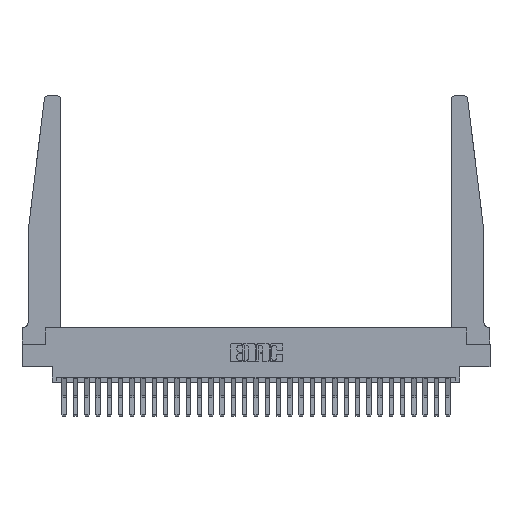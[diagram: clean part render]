
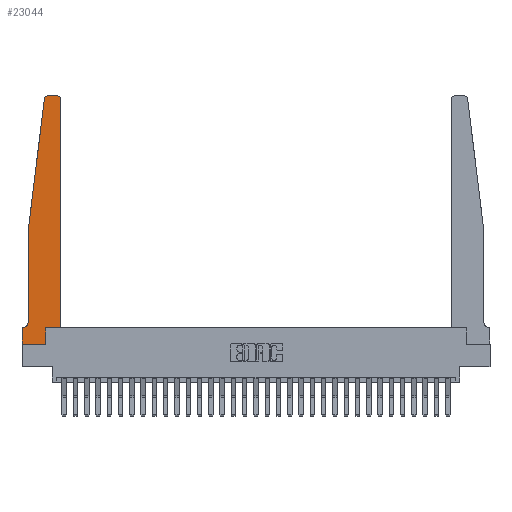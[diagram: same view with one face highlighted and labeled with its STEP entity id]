
A CAD part, top view. The second image highlights one B-rep face of the part: STEP entity #23044.
In plain terms, the highlighted planar face has unit normal (0, 0, 1).
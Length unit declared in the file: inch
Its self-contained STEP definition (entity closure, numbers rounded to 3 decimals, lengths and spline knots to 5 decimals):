
#455 = CARTESIAN_POINT ( 'NONE',  ( 0., 0., 0.37 ) ) ;
#739 = CARTESIAN_POINT ( 'NONE',  ( 0., 0., 0.37 ) ) ;
#849 = CIRCLE ( 'NONE', #28679, 0.05 ) ;
#1013 = DIRECTION ( 'NONE',  ( 0., 1., 0. ) ) ;
#1168 = VECTOR ( 'NONE', #25862, 39.37008 ) ;
#1215 = LINE ( 'NONE', #7613, #18985 ) ;
#1230 = AXIS2_PLACEMENT_3D ( 'NONE', #26266, #13032, #28503 ) ;
#1495 = LINE ( 'NONE', #10633, #19260 ) ;
#2930 = EDGE_CURVE ( 'NONE', #4829, #6440, #1495, .T. ) ;
#2967 = AXIS2_PLACEMENT_3D ( 'NONE', #22389, #9169, #24635 ) ;
#3096 = EDGE_CURVE ( 'NONE', #28401, #14144, #19587, .T. ) ;
#3815 = EDGE_CURVE ( 'NONE', #21683, #9113, #26487, .T. ) ;
#4109 = CARTESIAN_POINT ( 'NONE',  ( 0.24675, 2.72367, 0.37 ) ) ;
#4428 = VERTEX_POINT ( 'NONE', #26825 ) ;
#4437 = FACE_OUTER_BOUND ( 'NONE', #19238, .T. ) ;
#4468 = DIRECTION ( 'NONE',  ( 1., 0., 0. ) ) ;
#4701 = ORIENTED_EDGE ( 'NONE', *, *, #20294, .T. ) ;
#4829 = VERTEX_POINT ( 'NONE', #25830 ) ;
#4898 = DIRECTION ( 'NONE',  ( 0., -1., 0. ) ) ;
#4928 = ORIENTED_EDGE ( 'NONE', *, *, #7452, .T. ) ;
#5589 = ORIENTED_EDGE ( 'NONE', *, *, #7784, .T. ) ;
#5733 = CARTESIAN_POINT ( 'NONE',  ( 0.425, 2.72, 0.37 ) ) ;
#5795 = CIRCLE ( 'NONE', #2967, 0.03 ) ;
#5831 = CARTESIAN_POINT ( 'NONE',  ( 0.395, 2.75, 0.37 ) ) ;
#5966 = VECTOR ( 'NONE', #4898, 39.37008 ) ;
#6440 = VERTEX_POINT ( 'NONE', #20429 ) ;
#7452 = EDGE_CURVE ( 'NONE', #24324, #27096, #9694, .T. ) ;
#7613 = CARTESIAN_POINT ( 'NONE',  ( 0.065, 1.25, 0.37 ) ) ;
#7784 = EDGE_CURVE ( 'NONE', #4428, #20825, #1215, .T. ) ;
#8504 = DIRECTION ( 'NONE',  ( 1., 0., 0. ) ) ;
#9113 = VERTEX_POINT ( 'NONE', #16271 ) ;
#9169 = DIRECTION ( 'NONE',  ( 0., 0., 1. ) ) ;
#9309 = DIRECTION ( 'NONE',  ( 0., 1., 0. ) ) ;
#9577 = CARTESIAN_POINT ( 'NONE',  ( 0.015, 0.2375, 0.37 ) ) ;
#9694 = LINE ( 'NONE', #26305, #15561 ) ;
#10239 = AXIS2_PLACEMENT_3D ( 'NONE', #24108, #10910, #26341 ) ;
#10633 = CARTESIAN_POINT ( 'NONE',  ( 0.065, 0.1875, 0.37 ) ) ;
#10829 = PLANE ( 'NONE',  #1230 ) ;
#10910 = DIRECTION ( 'NONE',  ( 0., 0., 1. ) ) ;
#11789 = DIRECTION ( 'NONE',  ( -1., 0., 0. ) ) ;
#12186 = CARTESIAN_POINT ( 'NONE',  ( 0.425, 0.18, 0.37 ) ) ;
#12526 = CARTESIAN_POINT ( 'NONE',  ( 0.065, 1.25, 0.37 ) ) ;
#12924 = ORIENTED_EDGE ( 'NONE', *, *, #27746, .T. ) ;
#13032 = DIRECTION ( 'NONE',  ( 0., 0., 1. ) ) ;
#13515 = ORIENTED_EDGE ( 'NONE', *, *, #3815, .T. ) ;
#13750 = CARTESIAN_POINT ( 'NONE',  ( 0.065, 0.2375, 0.37 ) ) ;
#13751 = VECTOR ( 'NONE', #4468, 39.37008 ) ;
#13780 = LINE ( 'NONE', #12526, #1168 ) ;
#13911 = CARTESIAN_POINT ( 'NONE',  ( 0.2605, 0.18, 0.37 ) ) ;
#14144 = VERTEX_POINT ( 'NONE', #23072 ) ;
#14227 = DIRECTION ( 'NONE',  ( 0., -1., 0. ) ) ;
#14250 = ORIENTED_EDGE ( 'NONE', *, *, #3096, .T. ) ;
#14531 = LINE ( 'NONE', #12186, #20386 ) ;
#14820 = ORIENTED_EDGE ( 'NONE', *, *, #25143, .T. ) ;
#15411 = ORIENTED_EDGE ( 'NONE', *, *, #24760, .T. ) ;
#15548 = CARTESIAN_POINT ( 'NONE',  ( 0.425, 0.18, 0.37 ) ) ;
#15561 = VECTOR ( 'NONE', #8504, 39.37008 ) ;
#16009 = ORIENTED_EDGE ( 'NONE', *, *, #24220, .T. ) ;
#16186 = CARTESIAN_POINT ( 'NONE',  ( 0.2605, 0., 0.37 ) ) ;
#16271 = CARTESIAN_POINT ( 'NONE',  ( 0.27653, 2.75, 0.37 ) ) ;
#16910 = VECTOR ( 'NONE', #9309, 39.37008 ) ;
#17193 = EDGE_CURVE ( 'NONE', #20825, #4829, #849, .T. ) ;
#17734 = LINE ( 'NONE', #455, #5966 ) ;
#17862 = CARTESIAN_POINT ( 'NONE',  ( 0.25, 2.75, 0.37 ) ) ;
#18985 = VECTOR ( 'NONE', #14227, 39.37008 ) ;
#19238 = EDGE_LOOP ( 'NONE', ( #13515, #15411, #14820, #5589, #21778, #19929, #12924, #4928, #16009, #14250, #23189, #4701 ) ) ;
#19260 = VECTOR ( 'NONE', #25983, 39.37008 ) ;
#19501 = CIRCLE ( 'NONE', #10239, 0.03 ) ;
#19587 = LINE ( 'NONE', #15548, #13751 ) ;
#19929 = ORIENTED_EDGE ( 'NONE', *, *, #2930, .T. ) ;
#20294 = EDGE_CURVE ( 'NONE', #25081, #21683, #19501, .T. ) ;
#20386 = VECTOR ( 'NONE', #1013, 39.37008 ) ;
#20429 = CARTESIAN_POINT ( 'NONE',  ( 0., 0.1875, 0.37 ) ) ;
#20581 = VECTOR ( 'NONE', #26667, 39.37008 ) ;
#20825 = VERTEX_POINT ( 'NONE', #13750 ) ;
#21683 = VERTEX_POINT ( 'NONE', #5831 ) ;
#21778 = ORIENTED_EDGE ( 'NONE', *, *, #17193, .T. ) ;
#22389 = CARTESIAN_POINT ( 'NONE',  ( 0.27653, 2.72, 0.37 ) ) ;
#22821 = EDGE_CURVE ( 'NONE', #14144, #25081, #14531, .T. ) ;
#23044 = ADVANCED_FACE ( 'NONE', ( #4437 ), #10829, .T. ) ;
#23072 = CARTESIAN_POINT ( 'NONE',  ( 0.425, 0.18, 0.37 ) ) ;
#23189 = ORIENTED_EDGE ( 'NONE', *, *, #22821, .T. ) ;
#24108 = CARTESIAN_POINT ( 'NONE',  ( 0.395, 2.72, 0.37 ) ) ;
#24220 = EDGE_CURVE ( 'NONE', #27096, #28401, #27987, .T. ) ;
#24324 = VERTEX_POINT ( 'NONE', #739 ) ;
#24635 = DIRECTION ( 'NONE',  ( 1., 0., 0. ) ) ;
#24760 = EDGE_CURVE ( 'NONE', #9113, #25998, #5795, .T. ) ;
#24765 = CARTESIAN_POINT ( 'NONE',  ( 0.2605, 0.18, 0.37 ) ) ;
#25027 = DIRECTION ( 'NONE',  ( 0., 0., -1. ) ) ;
#25081 = VERTEX_POINT ( 'NONE', #5733 ) ;
#25143 = EDGE_CURVE ( 'NONE', #25998, #4428, #13780, .T. ) ;
#25830 = CARTESIAN_POINT ( 'NONE',  ( 0.015, 0.1875, 0.37 ) ) ;
#25862 = DIRECTION ( 'NONE',  ( -0.122, -0.992, 0. ) ) ;
#25983 = DIRECTION ( 'NONE',  ( -1., 0., 0. ) ) ;
#25998 = VERTEX_POINT ( 'NONE', #4109 ) ;
#26266 = CARTESIAN_POINT ( 'NONE',  ( 0., 0.1875, 0.37 ) ) ;
#26305 = CARTESIAN_POINT ( 'NONE',  ( 0., 0., 0.37 ) ) ;
#26341 = DIRECTION ( 'NONE',  ( 1., 0., 0. ) ) ;
#26487 = LINE ( 'NONE', #17862, #20581 ) ;
#26667 = DIRECTION ( 'NONE',  ( -1., 0., 0. ) ) ;
#26825 = CARTESIAN_POINT ( 'NONE',  ( 0.065, 1.25, 0.37 ) ) ;
#27096 = VERTEX_POINT ( 'NONE', #16186 ) ;
#27746 = EDGE_CURVE ( 'NONE', #6440, #24324, #17734, .T. ) ;
#27987 = LINE ( 'NONE', #24765, #16910 ) ;
#28401 = VERTEX_POINT ( 'NONE', #13911 ) ;
#28503 = DIRECTION ( 'NONE',  ( 1., 0., 0. ) ) ;
#28679 = AXIS2_PLACEMENT_3D ( 'NONE', #9577, #25027, #11789 ) ;
